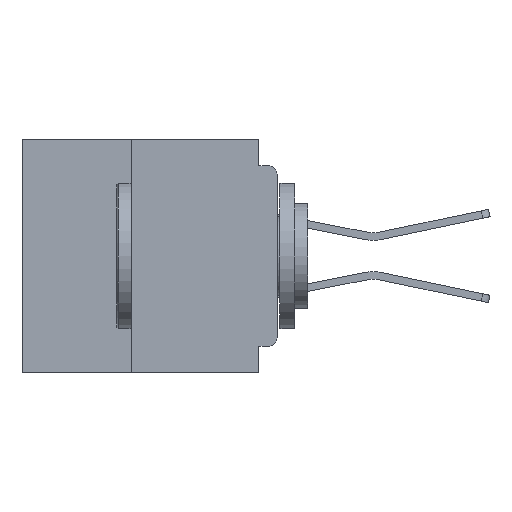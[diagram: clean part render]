
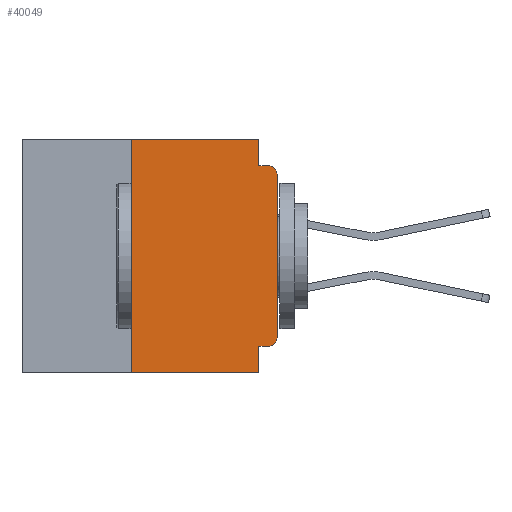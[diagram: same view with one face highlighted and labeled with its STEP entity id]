
A CAD part, left-side view. The second image highlights one B-rep face of the part: STEP entity #40049.
In plain terms, the highlighted planar face has unit normal (-1, 0, 0).
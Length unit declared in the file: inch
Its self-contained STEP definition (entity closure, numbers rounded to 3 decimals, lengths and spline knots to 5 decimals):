
#215 = CARTESIAN_POINT ( 'NONE',  ( 0., 0., -0.34 ) ) ;
#578 = PLANE ( 'NONE',  #19018 ) ;
#643 = CARTESIAN_POINT ( 'NONE',  ( 0., 0.437, -0.4 ) ) ;
#773 = EDGE_CURVE ( 'NONE', #11545, #4233, #3135, .T. ) ;
#1544 = EDGE_CURVE ( 'NONE', #21206, #15890, #30157, .T. ) ;
#1607 = CARTESIAN_POINT ( 'NONE',  ( 0., 0., -0.045 ) ) ;
#2040 = ORIENTED_EDGE ( 'NONE', *, *, #24229, .F. ) ;
#2514 = AXIS2_PLACEMENT_3D ( 'NONE', #19331, #44393, #22927 ) ;
#3135 = LINE ( 'NONE', #22910, #40232 ) ;
#3168 = CARTESIAN_POINT ( 'NONE',  ( 0., 0.015, -0.06 ) ) ;
#4233 = VERTEX_POINT ( 'NONE', #28705 ) ;
#4379 = DIRECTION ( 'NONE',  ( 0., -1., 0. ) ) ;
#4640 = CARTESIAN_POINT ( 'NONE',  ( 0., 0., 0. ) ) ;
#4705 = DIRECTION ( 'NONE',  ( 0., -1., 0. ) ) ;
#5108 = DIRECTION ( 'NONE',  ( 0., 0., -1. ) ) ;
#5446 = ORIENTED_EDGE ( 'NONE', *, *, #27439, .F. ) ;
#6775 = AXIS2_PLACEMENT_3D ( 'NONE', #3168, #28416, #6887 ) ;
#6887 = DIRECTION ( 'NONE',  ( 0., 0., -1. ) ) ;
#8282 = EDGE_CURVE ( 'NONE', #25594, #9491, #16367, .T. ) ;
#9399 = CARTESIAN_POINT ( 'NONE',  ( 0., 0.015, -0.045 ) ) ;
#9491 = VERTEX_POINT ( 'NONE', #215 ) ;
#11293 = VERTEX_POINT ( 'NONE', #32430 ) ;
#11545 = VERTEX_POINT ( 'NONE', #37516 ) ;
#11639 = CARTESIAN_POINT ( 'NONE',  ( 0., 0.437, 0. ) ) ;
#12388 = CARTESIAN_POINT ( 'NONE',  ( 0., 0.031, 0. ) ) ;
#12618 = LINE ( 'NONE', #12388, #19856 ) ;
#13013 = EDGE_CURVE ( 'NONE', #11293, #4233, #22001, .T. ) ;
#13577 = CARTESIAN_POINT ( 'NONE',  ( 0., 0.031, 0. ) ) ;
#14708 = CARTESIAN_POINT ( 'NONE',  ( 0., 0., -0.06 ) ) ;
#15027 = VECTOR ( 'NONE', #35265, 39.37008 ) ;
#15202 = DIRECTION ( 'NONE',  ( 0., 0., -1. ) ) ;
#15393 = EDGE_CURVE ( 'NONE', #11293, #33949, #16151, .T. ) ;
#15890 = VERTEX_POINT ( 'NONE', #9399 ) ;
#16151 = LINE ( 'NONE', #24447, #15027 ) ;
#16225 = EDGE_CURVE ( 'NONE', #33949, #21719, #19429, .T. ) ;
#16367 = CIRCLE ( 'NONE', #2514, 0.015 ) ;
#18268 = DIRECTION ( 'NONE',  ( 0., -1., 0. ) ) ;
#19018 = AXIS2_PLACEMENT_3D ( 'NONE', #11639, #36671, #15202 ) ;
#19106 = ORIENTED_EDGE ( 'NONE', *, *, #8282, .T. ) ;
#19213 = ORIENTED_EDGE ( 'NONE', *, *, #16225, .F. ) ;
#19222 = LINE ( 'NONE', #4640, #45576 ) ;
#19331 = CARTESIAN_POINT ( 'NONE',  ( 0., 0.015, -0.34 ) ) ;
#19419 = EDGE_CURVE ( 'NONE', #23072, #15890, #22017, .T. ) ;
#19429 = LINE ( 'NONE', #21867, #45772 ) ;
#19856 = VECTOR ( 'NONE', #5108, 39.37008 ) ;
#19963 = DIRECTION ( 'NONE',  ( 0., 1., 0. ) ) ;
#20141 = CARTESIAN_POINT ( 'NONE',  ( 0., 0.25, 0. ) ) ;
#21206 = VERTEX_POINT ( 'NONE', #28682 ) ;
#21719 = VERTEX_POINT ( 'NONE', #13577 ) ;
#21867 = CARTESIAN_POINT ( 'NONE',  ( 0., 0.437, 0. ) ) ;
#22001 = LINE ( 'NONE', #643, #39895 ) ;
#22017 = CIRCLE ( 'NONE', #6775, 0.015 ) ;
#22239 = EDGE_LOOP ( 'NONE', ( #41455, #45912, #25908, #5446, #19213, #24202, #25518, #25192, #2040, #19106 ) ) ;
#22910 = CARTESIAN_POINT ( 'NONE',  ( 0., 0.031, -0.4 ) ) ;
#22927 = DIRECTION ( 'NONE',  ( 0., 0., -1. ) ) ;
#23061 = DIRECTION ( 'NONE',  ( 0., 0., -1. ) ) ;
#23072 = VERTEX_POINT ( 'NONE', #14708 ) ;
#24202 = ORIENTED_EDGE ( 'NONE', *, *, #15393, .F. ) ;
#24229 = EDGE_CURVE ( 'NONE', #25594, #11545, #44857, .T. ) ;
#24447 = CARTESIAN_POINT ( 'NONE',  ( 0., 0.25, -0.4 ) ) ;
#25192 = ORIENTED_EDGE ( 'NONE', *, *, #773, .F. ) ;
#25518 = ORIENTED_EDGE ( 'NONE', *, *, #13013, .T. ) ;
#25594 = VERTEX_POINT ( 'NONE', #27735 ) ;
#25810 = VECTOR ( 'NONE', #19963, 39.37008 ) ;
#25908 = ORIENTED_EDGE ( 'NONE', *, *, #1544, .F. ) ;
#27439 = EDGE_CURVE ( 'NONE', #21719, #21206, #12618, .T. ) ;
#27735 = CARTESIAN_POINT ( 'NONE',  ( 0., 0.015, -0.355 ) ) ;
#28416 = DIRECTION ( 'NONE',  ( -1., 0., 0. ) ) ;
#28682 = CARTESIAN_POINT ( 'NONE',  ( 0., 0.031, -0.045 ) ) ;
#28705 = CARTESIAN_POINT ( 'NONE',  ( 0., 0.031, -0.4 ) ) ;
#30157 = LINE ( 'NONE', #1607, #39605 ) ;
#32430 = CARTESIAN_POINT ( 'NONE',  ( 0., 0.25, -0.4 ) ) ;
#33399 = DIRECTION ( 'NONE',  ( 0., 0., 1. ) ) ;
#33949 = VERTEX_POINT ( 'NONE', #20141 ) ;
#35265 = DIRECTION ( 'NONE',  ( 0., 0., 1. ) ) ;
#36671 = DIRECTION ( 'NONE',  ( 1., 0., 0. ) ) ;
#37163 = FACE_OUTER_BOUND ( 'NONE', #22239, .T. ) ;
#37516 = CARTESIAN_POINT ( 'NONE',  ( 0., 0.031, -0.355 ) ) ;
#39605 = VECTOR ( 'NONE', #4705, 39.37008 ) ;
#39895 = VECTOR ( 'NONE', #4379, 39.37008 ) ;
#40049 = ADVANCED_FACE ( 'NONE', ( #37163 ), #578, .F. ) ;
#40123 = EDGE_CURVE ( 'NONE', #9491, #23072, #19222, .T. ) ;
#40232 = VECTOR ( 'NONE', #23061, 39.37008 ) ;
#41455 = ORIENTED_EDGE ( 'NONE', *, *, #40123, .T. ) ;
#44393 = DIRECTION ( 'NONE',  ( -1., 0., 0. ) ) ;
#44857 = LINE ( 'NONE', #45042, #25810 ) ;
#45042 = CARTESIAN_POINT ( 'NONE',  ( 0., 0., -0.355 ) ) ;
#45576 = VECTOR ( 'NONE', #33399, 39.37008 ) ;
#45772 = VECTOR ( 'NONE', #18268, 39.37008 ) ;
#45912 = ORIENTED_EDGE ( 'NONE', *, *, #19419, .T. ) ;
